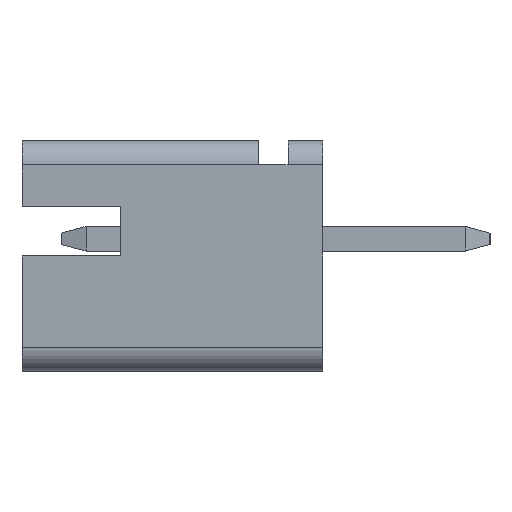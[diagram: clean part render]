
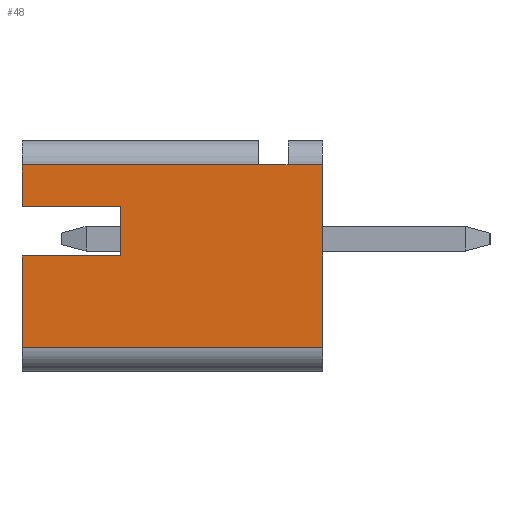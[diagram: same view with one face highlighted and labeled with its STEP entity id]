
A CAD part, left-side view. The second image highlights one B-rep face of the part: STEP entity #48.
In plain terms, the highlighted planar face has unit normal (-1, 0, 0).
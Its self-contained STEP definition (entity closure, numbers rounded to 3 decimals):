
#48 = ADVANCED_FACE ( 'NONE', ( #3458 ), #2444, .F. ) ;
#49 = VECTOR ( 'NONE', #3486, 1000. ) ;
#243 = VERTEX_POINT ( 'NONE', #1458 ) ;
#268 = EDGE_CURVE ( 'NONE', #2089, #4149, #3972, .T. ) ;
#452 = EDGE_CURVE ( 'NONE', #2990, #3296, #3236, .T. ) ;
#536 = VERTEX_POINT ( 'NONE', #2057 ) ;
#564 = VERTEX_POINT ( 'NONE', #3916 ) ;
#594 = VECTOR ( 'NONE', #2517, 1000. ) ;
#604 = VECTOR ( 'NONE', #4533, 1000. ) ;
#635 = DIRECTION ( 'NONE',  ( 0., 0., -1. ) ) ;
#656 = CARTESIAN_POINT ( 'NONE',  ( -2., 0., 0. ) ) ;
#751 = CARTESIAN_POINT ( 'NONE',  ( -2., 0., 2. ) ) ;
#864 = EDGE_CURVE ( 'NONE', #4294, #3296, #1884, .T. ) ;
#915 = ORIENTED_EDGE ( 'NONE', *, *, #1515, .F. ) ;
#984 = EDGE_CURVE ( 'NONE', #4185, #536, #2438, .T. ) ;
#1085 = CARTESIAN_POINT ( 'NONE',  ( -2., 6.1, 1.5 ) ) ;
#1198 = ORIENTED_EDGE ( 'NONE', *, *, #1540, .F. ) ;
#1217 = VECTOR ( 'NONE', #1450, 1000. ) ;
#1236 = ORIENTED_EDGE ( 'NONE', *, *, #2227, .T. ) ;
#1327 = LINE ( 'NONE', #2760, #3804 ) ;
#1344 = CARTESIAN_POINT ( 'NONE',  ( -2., 4.1, -0.35 ) ) ;
#1345 = LINE ( 'NONE', #3853, #2023 ) ;
#1427 = CARTESIAN_POINT ( 'NONE',  ( -2., 1.3, 1.5 ) ) ;
#1450 = DIRECTION ( 'NONE',  ( 0., -1., 0. ) ) ;
#1458 = CARTESIAN_POINT ( 'NONE',  ( -2., 6.1, 0.65 ) ) ;
#1515 = EDGE_CURVE ( 'NONE', #4149, #564, #3504, .T. ) ;
#1540 = EDGE_CURVE ( 'NONE', #2990, #2089, #4049, .T. ) ;
#1552 = CARTESIAN_POINT ( 'NONE',  ( -2., 6.1, -0.35 ) ) ;
#1557 = VERTEX_POINT ( 'NONE', #1085 ) ;
#1623 = ORIENTED_EDGE ( 'NONE', *, *, #268, .F. ) ;
#1796 = DIRECTION ( 'NONE',  ( 0., 1., 0. ) ) ;
#1868 = EDGE_CURVE ( 'NONE', #4185, #1557, #1327, .T. ) ;
#1884 = LINE ( 'NONE', #751, #3538 ) ;
#2010 = CARTESIAN_POINT ( 'NONE',  ( -2., 1.3, 1.5 ) ) ;
#2023 = VECTOR ( 'NONE', #3198, 1000. ) ;
#2057 = CARTESIAN_POINT ( 'NONE',  ( -2., 0.7, 1.5 ) ) ;
#2088 = VECTOR ( 'NONE', #3893, 1000. ) ;
#2089 = VERTEX_POINT ( 'NONE', #1552 ) ;
#2142 = AXIS2_PLACEMENT_3D ( 'NONE', #656, #2778, #635 ) ;
#2227 = EDGE_CURVE ( 'NONE', #4294, #536, #3876, .T. ) ;
#2257 = EDGE_CURVE ( 'NONE', #243, #1557, #1345, .T. ) ;
#2260 = CARTESIAN_POINT ( 'NONE',  ( -2., 6.1, -0.35 ) ) ;
#2414 = CARTESIAN_POINT ( 'NONE',  ( -2., 0., -2.2 ) ) ;
#2438 = LINE ( 'NONE', #1427, #1217 ) ;
#2444 = PLANE ( 'NONE',  #2142 ) ;
#2517 = DIRECTION ( 'NONE',  ( 0., -1., 0. ) ) ;
#2519 = ORIENTED_EDGE ( 'NONE', *, *, #864, .F. ) ;
#2760 = CARTESIAN_POINT ( 'NONE',  ( -2., 0., 1.5 ) ) ;
#2778 = DIRECTION ( 'NONE',  ( 1., 0., 0. ) ) ;
#2785 = CARTESIAN_POINT ( 'NONE',  ( -2., 4.1, 0.65 ) ) ;
#2791 = ORIENTED_EDGE ( 'NONE', *, *, #3530, .F. ) ;
#2990 = VERTEX_POINT ( 'NONE', #4021 ) ;
#3038 = ORIENTED_EDGE ( 'NONE', *, *, #1868, .T. ) ;
#3110 = CARTESIAN_POINT ( 'NONE',  ( -2., 0., 1.5 ) ) ;
#3198 = DIRECTION ( 'NONE',  ( 0., 0., 1. ) ) ;
#3236 = LINE ( 'NONE', #2414, #2088 ) ;
#3254 = DIRECTION ( 'NONE',  ( 0., 0., 1. ) ) ;
#3296 = VERTEX_POINT ( 'NONE', #4409 ) ;
#3399 = ORIENTED_EDGE ( 'NONE', *, *, #2257, .F. ) ;
#3422 = LINE ( 'NONE', #4285, #4570 ) ;
#3458 = FACE_OUTER_BOUND ( 'NONE', #4534, .T. ) ;
#3486 = DIRECTION ( 'NONE',  ( 0., 0., 1. ) ) ;
#3504 = LINE ( 'NONE', #2785, #49 ) ;
#3530 = EDGE_CURVE ( 'NONE', #564, #243, #3422, .T. ) ;
#3538 = VECTOR ( 'NONE', #4303, 1000. ) ;
#3610 = ORIENTED_EDGE ( 'NONE', *, *, #984, .F. ) ;
#3804 = VECTOR ( 'NONE', #4188, 1000. ) ;
#3853 = CARTESIAN_POINT ( 'NONE',  ( -2., 6.1, 2. ) ) ;
#3876 = LINE ( 'NONE', #3110, #604 ) ;
#3877 = VECTOR ( 'NONE', #3254, 1000. ) ;
#3893 = DIRECTION ( 'NONE',  ( 0., -1., 0. ) ) ;
#3916 = CARTESIAN_POINT ( 'NONE',  ( -2., 4.1, 0.65 ) ) ;
#3972 = LINE ( 'NONE', #4319, #594 ) ;
#4021 = CARTESIAN_POINT ( 'NONE',  ( -2., 6.1, -2.2 ) ) ;
#4049 = LINE ( 'NONE', #2260, #3877 ) ;
#4149 = VERTEX_POINT ( 'NONE', #1344 ) ;
#4178 = CARTESIAN_POINT ( 'NONE',  ( -2., 0., 1.5 ) ) ;
#4185 = VERTEX_POINT ( 'NONE', #2010 ) ;
#4188 = DIRECTION ( 'NONE',  ( 0., 1., 0. ) ) ;
#4285 = CARTESIAN_POINT ( 'NONE',  ( -2., 6.1, 0.65 ) ) ;
#4294 = VERTEX_POINT ( 'NONE', #4178 ) ;
#4303 = DIRECTION ( 'NONE',  ( 0., 0., -1. ) ) ;
#4319 = CARTESIAN_POINT ( 'NONE',  ( -2., 6.1, -0.35 ) ) ;
#4409 = CARTESIAN_POINT ( 'NONE',  ( -2., 0., -2.2 ) ) ;
#4533 = DIRECTION ( 'NONE',  ( 0., 1., 0. ) ) ;
#4534 = EDGE_LOOP ( 'NONE', ( #1198, #4561, #2519, #1236, #3610, #3038, #3399, #2791, #915, #1623 ) ) ;
#4561 = ORIENTED_EDGE ( 'NONE', *, *, #452, .T. ) ;
#4570 = VECTOR ( 'NONE', #1796, 1000. ) ;
